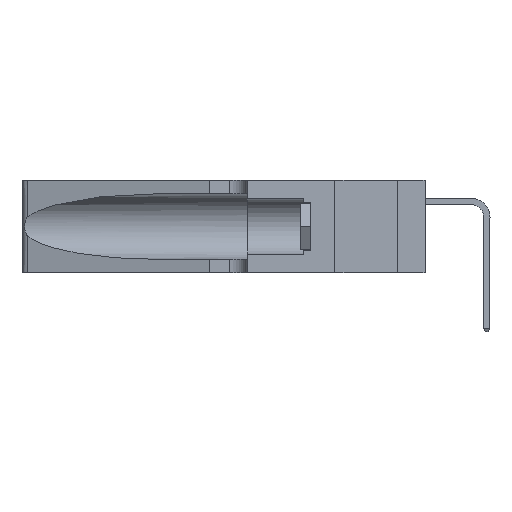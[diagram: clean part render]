
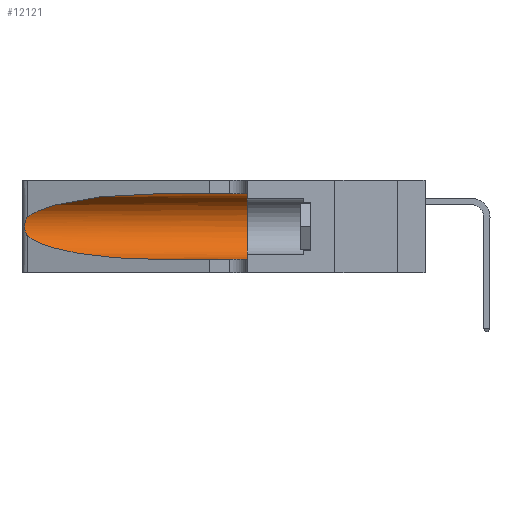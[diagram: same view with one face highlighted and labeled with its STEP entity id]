
A CAD part, left-side view. The second image highlights one B-rep face of the part: STEP entity #12121.
In plain terms, the highlighted cylindrical face has radius 3.308 mm (diameter 6.617 mm), a partial arc.
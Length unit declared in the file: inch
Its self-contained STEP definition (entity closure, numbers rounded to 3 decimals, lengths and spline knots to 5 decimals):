
#176 = VECTOR ( 'NONE', #30565, 39.37008 ) ;
#177 = CARTESIAN_POINT ( 'NONE',  ( 0.1305, 0.72297, 0.05475 ) ) ;
#673 = CARTESIAN_POINT ( 'NONE',  ( 0.25487, 1.22718, 0.14631 ) ) ;
#1568 = CARTESIAN_POINT ( 'NONE',  ( 0.1305, 0.72297, 0.31525 ) ) ;
#2103 = CARTESIAN_POINT ( 'NONE',  ( 0.26075, 1.23896, 0.178 ) ) ;
#2591 = ORIENTED_EDGE ( 'NONE', *, *, #34374, .T. ) ;
#3221 = VECTOR ( 'NONE', #27776, 39.37008 ) ;
#3333 = AXIS2_PLACEMENT_3D ( 'NONE', #30747, #12988, #9999 ) ;
#3746 = EDGE_CURVE ( 'NONE', #15847, #37464, #33864, .T. ) ;
#3942 = FACE_OUTER_BOUND ( 'NONE', #28778, .T. ) ;
#4470 = CARTESIAN_POINT ( 'NONE',  ( 0.1305, 0.72297, 0.31525 ) ) ;
#4586 = CARTESIAN_POINT ( 'NONE',  ( 0.18966, 0.96281, 0.31525 ) ) ;
#5108 = CARTESIAN_POINT ( 'NONE',  ( 0.25856, 1.23593, 0.16098 ) ) ;
#5287 = VERTEX_POINT ( 'NONE', #25710 ) ;
#6222 = B_SPLINE_CURVE_WITH_KNOTS ( 'NONE', 3,
 ( #28734, #31700, #13942, #34676, #16896, #37639, #19846, #2103, #22859, #5108, #25865, #8097, #28860, #11084 ),
 .UNSPECIFIED., .F., .F.,
 ( 4, 2, 2, 2, 2, 2, 4 ),
 ( 0., 0.00027, 0.00053, 0.00107, 0.0016, 0.00187, 0.00214 ),
 .UNSPECIFIED. ) ;
#6337 = ORIENTED_EDGE ( 'NONE', *, *, #18899, .T. ) ;
#7011 = CARTESIAN_POINT ( 'NONE',  ( 0.1305, 1.61858, 0.31525 ) ) ;
#7585 = CARTESIAN_POINT ( 'NONE',  ( 0.2373, 1.15595, 0.28018 ) ) ;
#8097 = CARTESIAN_POINT ( 'NONE',  ( 0.25639, 1.23186, 0.15144 ) ) ;
#8101 = ORIENTED_EDGE ( 'NONE', *, *, #3746, .F. ) ;
#8734 = CARTESIAN_POINT ( 'NONE',  ( 0.1305, 0.72297, 0.05475 ) ) ;
#9462 = EDGE_CURVE ( 'NONE', #20211, #27491, #22807, .T. ) ;
#9642 = CIRCLE ( 'NONE', #33367, 0.13025 ) ;
#9817 = CARTESIAN_POINT ( 'NONE',  ( 0.1305, 1.61858, 0.05475 ) ) ;
#9999 = DIRECTION ( 'NONE',  ( 0., 0., -1. ) ) ;
#10932 = CYLINDRICAL_SURFACE ( 'NONE', #3333, 0.13025 ) ;
#11084 = CARTESIAN_POINT ( 'NONE',  ( 0.25487, 1.22718, 0.14631 ) ) ;
#12121 = ADVANCED_FACE ( 'NONE', ( #3942 ), #10932, .F. ) ;
#12903 = ORIENTED_EDGE ( 'NONE', *, *, #27520, .F. ) ;
#12988 = DIRECTION ( 'NONE',  ( 0., -1., 0. ) ) ;
#13942 = CARTESIAN_POINT ( 'NONE',  ( 0.25639, 1.23184, 0.21858 ) ) ;
#15105 = CARTESIAN_POINT ( 'NONE',  ( 0.2373, 1.15595, 0.08982 ) ) ;
#15847 = VERTEX_POINT ( 'NONE', #4470 ) ;
#16896 = CARTESIAN_POINT ( 'NONE',  ( 0.25854, 1.2359, 0.20912 ) ) ;
#16900 = CARTESIAN_POINT ( 'NONE',  ( 0.1305, 0.35, 0.05475 ) ) ;
#17007 = LINE ( 'NONE', #9817, #176 ) ;
#17770 = DIRECTION ( 'NONE',  ( 0., 1., 0. ) ) ;
#18059 = CARTESIAN_POINT ( 'NONE',  ( 0.18966, 0.96281, 0.05475 ) ) ;
#18899 = EDGE_CURVE ( 'NONE', #27491, #25108, #17007, .T. ) ;
#19846 = CARTESIAN_POINT ( 'NONE',  ( 0.26075, 1.23896, 0.19203 ) ) ;
#20211 = VERTEX_POINT ( 'NONE', #673 ) ;
#20803 = ORIENTED_EDGE ( 'NONE', *, *, #9462, .T. ) ;
#22807 =( BOUNDED_CURVE ( )  B_SPLINE_CURVE ( 3, ( #35839, #15105, #18059, #177 ),
 .UNSPECIFIED., .F., .F. ) 
 B_SPLINE_CURVE_WITH_KNOTS ( ( 4, 4 ),
 ( 3.44316, 4.71239 ),
 .UNSPECIFIED. ) 
 CURVE ( )  GEOMETRIC_REPRESENTATION_ITEM ( )  RATIONAL_B_SPLINE_CURVE ( ( 1., 0.87, 0.87, 1. ) ) 
 REPRESENTATION_ITEM ( '' )  );
#22859 = CARTESIAN_POINT ( 'NONE',  ( 0.26017, 1.23833, 0.17102 ) ) ;
#25108 = VERTEX_POINT ( 'NONE', #16900 ) ;
#25710 = CARTESIAN_POINT ( 'NONE',  ( 0.25487, 1.22718, 0.22369 ) ) ;
#25865 = CARTESIAN_POINT ( 'NONE',  ( 0.25789, 1.23486, 0.15765 ) ) ;
#26168 =( BOUNDED_CURVE ( )  B_SPLINE_CURVE ( 3, ( #1568, #4586, #7585, #28341 ),
 .UNSPECIFIED., .F., .T. ) 
 B_SPLINE_CURVE_WITH_KNOTS ( ( 4, 4 ),
 ( 1.5708, 2.84003 ),
 .UNSPECIFIED. ) 
 CURVE ( )  GEOMETRIC_REPRESENTATION_ITEM ( )  RATIONAL_B_SPLINE_CURVE ( ( 1., 0.87, 0.87, 1. ) ) 
 REPRESENTATION_ITEM ( '' )  );
#27491 = VERTEX_POINT ( 'NONE', #8734 ) ;
#27520 = EDGE_CURVE ( 'NONE', #37464, #25108, #9642, .T. ) ;
#27776 = DIRECTION ( 'NONE',  ( 0., -1., 0. ) ) ;
#28341 = CARTESIAN_POINT ( 'NONE',  ( 0.25487, 1.22718, 0.22369 ) ) ;
#28734 = CARTESIAN_POINT ( 'NONE',  ( 0.25487, 1.22718, 0.22369 ) ) ;
#28778 = EDGE_LOOP ( 'NONE', ( #2591, #30703, #20803, #6337, #12903, #8101 ) ) ;
#28860 = CARTESIAN_POINT ( 'NONE',  ( 0.25555, 1.22993, 0.14849 ) ) ;
#30565 = DIRECTION ( 'NONE',  ( 0., -1., 0. ) ) ;
#30703 = ORIENTED_EDGE ( 'NONE', *, *, #37318, .T. ) ;
#30747 = CARTESIAN_POINT ( 'NONE',  ( 0.1305, 1.61858, 0.185 ) ) ;
#31700 = CARTESIAN_POINT ( 'NONE',  ( 0.25555, 1.22994, 0.2215 ) ) ;
#33367 = AXIS2_PLACEMENT_3D ( 'NONE', #35562, #17770, #38534 ) ;
#33864 = LINE ( 'NONE', #7011, #3221 ) ;
#34374 = EDGE_CURVE ( 'NONE', #15847, #5287, #26168, .T. ) ;
#34676 = CARTESIAN_POINT ( 'NONE',  ( 0.25787, 1.23484, 0.2124 ) ) ;
#35562 = CARTESIAN_POINT ( 'NONE',  ( 0.1305, 0.35, 0.185 ) ) ;
#35839 = CARTESIAN_POINT ( 'NONE',  ( 0.25487, 1.22718, 0.14631 ) ) ;
#37318 = EDGE_CURVE ( 'NONE', #5287, #20211, #6222, .T. ) ;
#37464 = VERTEX_POINT ( 'NONE', #38280 ) ;
#37639 = CARTESIAN_POINT ( 'NONE',  ( 0.26018, 1.23835, 0.19895 ) ) ;
#38280 = CARTESIAN_POINT ( 'NONE',  ( 0.1305, 0.35, 0.31525 ) ) ;
#38534 = DIRECTION ( 'NONE',  ( 0., 0., 1. ) ) ;
